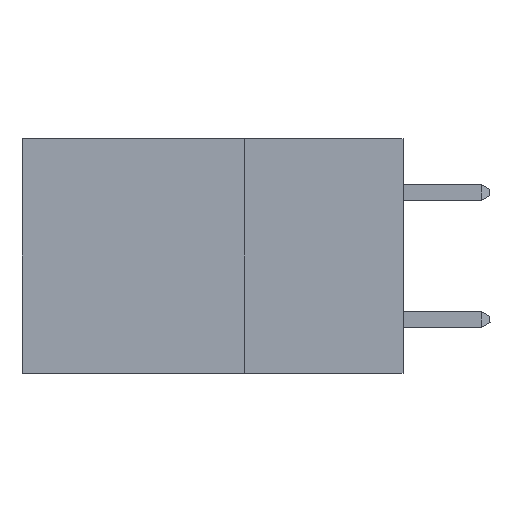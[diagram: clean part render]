
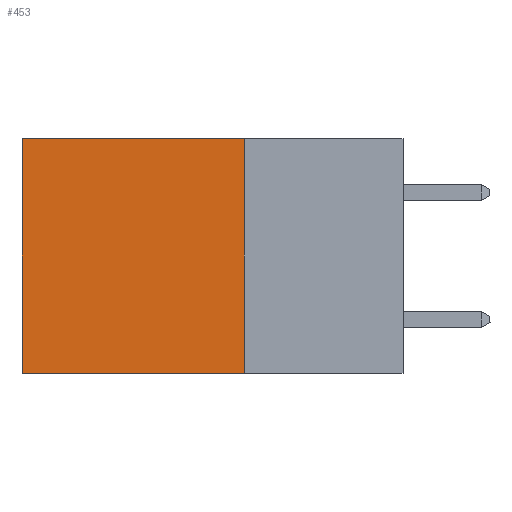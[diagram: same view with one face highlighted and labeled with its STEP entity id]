
A CAD part, left-side view. The second image highlights one B-rep face of the part: STEP entity #453.
In plain terms, the highlighted planar face has unit normal (-1, 0, 0).
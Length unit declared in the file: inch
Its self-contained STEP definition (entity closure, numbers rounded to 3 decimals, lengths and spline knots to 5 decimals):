
#453 = ADVANCED_FACE ( 'NONE', ( #26247 ), #5587, .F. ) ;
#844 = EDGE_CURVE ( 'NONE', #8039, #11865, #6780, .T. ) ;
#2029 = DIRECTION ( 'NONE',  ( 1., 0., 0. ) ) ;
#2749 = ORIENTED_EDGE ( 'NONE', *, *, #10411, .F. ) ;
#3059 = EDGE_CURVE ( 'NONE', #25497, #11683, #18497, .T. ) ;
#3349 = CARTESIAN_POINT ( 'NONE',  ( 0.2875, 0.25, 0. ) ) ;
#3866 = CARTESIAN_POINT ( 'NONE',  ( 0.2875, 0.6, -0.37 ) ) ;
#4651 = LINE ( 'NONE', #6550, #6532 ) ;
#4750 = EDGE_CURVE ( 'NONE', #11683, #11865, #26286, .T. ) ;
#5587 = PLANE ( 'NONE',  #19098 ) ;
#5744 = EDGE_LOOP ( 'NONE', ( #25570, #20930, #2749, #22920 ) ) ;
#5823 = CARTESIAN_POINT ( 'NONE',  ( 0.2875, 0.25, -0.37 ) ) ;
#6532 = VECTOR ( 'NONE', #16466, 39.37008 ) ;
#6550 = CARTESIAN_POINT ( 'NONE',  ( 0.2875, 0.25, 0. ) ) ;
#6780 = LINE ( 'NONE', #8845, #8059 ) ;
#7327 = DIRECTION ( 'NONE',  ( 0., 1., 0. ) ) ;
#8039 = VERTEX_POINT ( 'NONE', #5823 ) ;
#8059 = VECTOR ( 'NONE', #8549, 39.37008 ) ;
#8549 = DIRECTION ( 'NONE',  ( 0., 1., 0. ) ) ;
#8845 = CARTESIAN_POINT ( 'NONE',  ( 0.2875, 0.25, -0.37 ) ) ;
#10411 = EDGE_CURVE ( 'NONE', #25497, #8039, #4651, .T. ) ;
#10669 = CARTESIAN_POINT ( 'NONE',  ( 0.2875, 0.6, 0. ) ) ;
#11683 = VERTEX_POINT ( 'NONE', #10669 ) ;
#11865 = VERTEX_POINT ( 'NONE', #3866 ) ;
#14413 = DIRECTION ( 'NONE',  ( 0., 0., -1. ) ) ;
#16108 = VECTOR ( 'NONE', #24138, 39.37008 ) ;
#16466 = DIRECTION ( 'NONE',  ( 0., 0., -1. ) ) ;
#18136 = CARTESIAN_POINT ( 'NONE',  ( 0.2875, 0.6, 0. ) ) ;
#18497 = LINE ( 'NONE', #3349, #25429 ) ;
#19098 = AXIS2_PLACEMENT_3D ( 'NONE', #22324, #2029, #14413 ) ;
#19868 = CARTESIAN_POINT ( 'NONE',  ( 0.2875, 0.25, 0. ) ) ;
#20930 = ORIENTED_EDGE ( 'NONE', *, *, #844, .F. ) ;
#22324 = CARTESIAN_POINT ( 'NONE',  ( 0.2875, 0.25, 0. ) ) ;
#22920 = ORIENTED_EDGE ( 'NONE', *, *, #3059, .T. ) ;
#24138 = DIRECTION ( 'NONE',  ( 0., 0., -1. ) ) ;
#25429 = VECTOR ( 'NONE', #7327, 39.37008 ) ;
#25497 = VERTEX_POINT ( 'NONE', #19868 ) ;
#25570 = ORIENTED_EDGE ( 'NONE', *, *, #4750, .T. ) ;
#26247 = FACE_OUTER_BOUND ( 'NONE', #5744, .T. ) ;
#26286 = LINE ( 'NONE', #18136, #16108 ) ;
